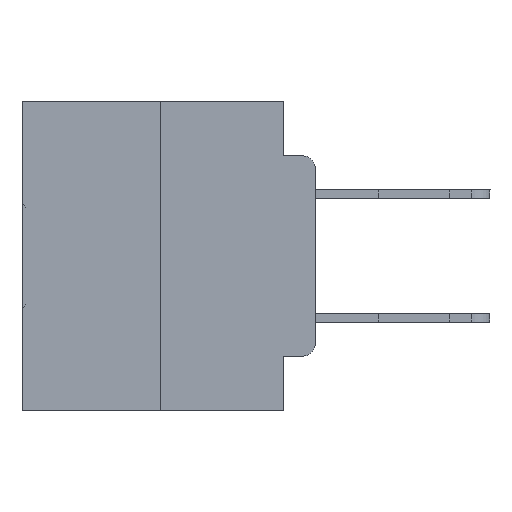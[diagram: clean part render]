
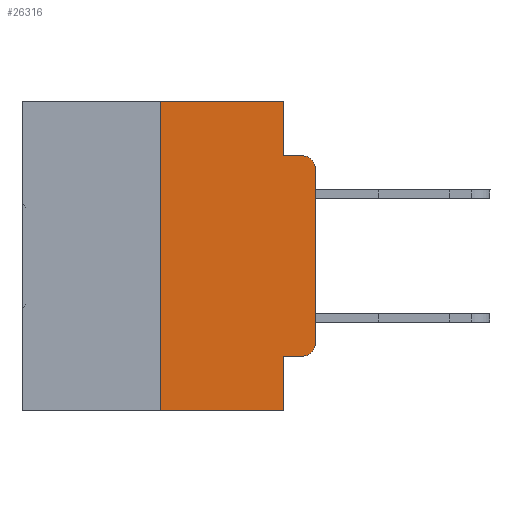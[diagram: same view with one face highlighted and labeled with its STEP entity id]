
A CAD part, left-side view. The second image highlights one B-rep face of the part: STEP entity #26316.
In plain terms, the highlighted planar face has unit normal (-1, 0, 0).
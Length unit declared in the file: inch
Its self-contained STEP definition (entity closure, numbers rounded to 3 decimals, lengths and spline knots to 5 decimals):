
#191 = ORIENTED_EDGE ( 'NONE', *, *, #10974, .T. ) ;
#328 = EDGE_CURVE ( 'NONE', #5537, #6284, #32345, .T. ) ;
#333 = ORIENTED_EDGE ( 'NONE', *, *, #328, .F. ) ;
#639 = CARTESIAN_POINT ( 'NONE',  ( 0., 0., 0. ) ) ;
#1246 = VECTOR ( 'NONE', #32396, 39.37008 ) ;
#1451 = EDGE_CURVE ( 'NONE', #7084, #6441, #4992, .T. ) ;
#1473 = CARTESIAN_POINT ( 'NONE',  ( 0., 0.051, -0.4115 ) ) ;
#1488 = EDGE_CURVE ( 'NONE', #19117, #7084, #26306, .T. ) ;
#1860 = LINE ( 'NONE', #32029, #22420 ) ;
#2245 = VECTOR ( 'NONE', #16539, 39.37008 ) ;
#3180 = DIRECTION ( 'NONE',  ( 0., 0., -1. ) ) ;
#4992 = LINE ( 'NONE', #639, #22798 ) ;
#5026 = EDGE_CURVE ( 'NONE', #6441, #25924, #17452, .T. ) ;
#5537 = VERTEX_POINT ( 'NONE', #14257 ) ;
#5823 = DIRECTION ( 'NONE',  ( 0., 0., 1. ) ) ;
#5964 = LINE ( 'NONE', #24060, #26525 ) ;
#6284 = VERTEX_POINT ( 'NONE', #23575 ) ;
#6441 = VERTEX_POINT ( 'NONE', #29427 ) ;
#6510 = CARTESIAN_POINT ( 'NONE',  ( 0., 0.051, 0. ) ) ;
#7084 = VERTEX_POINT ( 'NONE', #23832 ) ;
#7607 = FACE_OUTER_BOUND ( 'NONE', #13161, .T. ) ;
#7897 = DIRECTION ( 'NONE',  ( 0., -1., 0. ) ) ;
#8152 = CARTESIAN_POINT ( 'NONE',  ( 0., 0.02, -0.3915 ) ) ;
#9524 = DIRECTION ( 'NONE',  ( 0., 0., -1. ) ) ;
#10262 = ORIENTED_EDGE ( 'NONE', *, *, #20951, .T. ) ;
#10974 = EDGE_CURVE ( 'NONE', #5537, #23899, #1860, .T. ) ;
#12241 = VECTOR ( 'NONE', #24153, 39.37008 ) ;
#12527 = LINE ( 'NONE', #1473, #2245 ) ;
#12942 = AXIS2_PLACEMENT_3D ( 'NONE', #8152, #18645, #16030 ) ;
#13098 = ORIENTED_EDGE ( 'NONE', *, *, #5026, .T. ) ;
#13161 = EDGE_LOOP ( 'NONE', ( #13974, #13098, #29983, #25853, #30564, #333, #191, #24889, #10262, #20407 ) ) ;
#13367 = CARTESIAN_POINT ( 'NONE',  ( 0., 0.473, 0. ) ) ;
#13407 = AXIS2_PLACEMENT_3D ( 'NONE', #13367, #25927, #3180 ) ;
#13681 = VERTEX_POINT ( 'NONE', #15306 ) ;
#13692 = PLANE ( 'NONE',  #13407 ) ;
#13974 = ORIENTED_EDGE ( 'NONE', *, *, #1451, .T. ) ;
#14257 = CARTESIAN_POINT ( 'NONE',  ( 0., 0.25, -0.5 ) ) ;
#14333 = CARTESIAN_POINT ( 'NONE',  ( 0., 0.02, -0.4115 ) ) ;
#15172 = CARTESIAN_POINT ( 'NONE',  ( 0., 0.051, -0.0885 ) ) ;
#15306 = CARTESIAN_POINT ( 'NONE',  ( 0., 0.051, -0.4115 ) ) ;
#15816 = VERTEX_POINT ( 'NONE', #6510 ) ;
#16030 = DIRECTION ( 'NONE',  ( 0., 0., -1. ) ) ;
#16056 = LINE ( 'NONE', #23054, #20396 ) ;
#16539 = DIRECTION ( 'NONE',  ( 0., -1., 0. ) ) ;
#17262 = EDGE_CURVE ( 'NONE', #6284, #15816, #23765, .T. ) ;
#17452 = CIRCLE ( 'NONE', #23600, 0.02 ) ;
#17694 = EDGE_CURVE ( 'NONE', #13681, #23899, #5964, .T. ) ;
#17931 = CARTESIAN_POINT ( 'NONE',  ( 0., 0.051, -0.5 ) ) ;
#17984 = VERTEX_POINT ( 'NONE', #15172 ) ;
#18645 = DIRECTION ( 'NONE',  ( -1., 0., 0. ) ) ;
#18948 = LINE ( 'NONE', #31442, #12241 ) ;
#19117 = VERTEX_POINT ( 'NONE', #14333 ) ;
#19669 = CARTESIAN_POINT ( 'NONE',  ( 0., 0.02, -0.0885 ) ) ;
#20396 = VECTOR ( 'NONE', #7897, 39.37008 ) ;
#20407 = ORIENTED_EDGE ( 'NONE', *, *, #1488, .T. ) ;
#20951 = EDGE_CURVE ( 'NONE', #13681, #19117, #12527, .T. ) ;
#20970 = DIRECTION ( 'NONE',  ( 0., 0., 1. ) ) ;
#22317 = EDGE_CURVE ( 'NONE', #15816, #17984, #18948, .T. ) ;
#22420 = VECTOR ( 'NONE', #29818, 39.37008 ) ;
#22798 = VECTOR ( 'NONE', #5823, 39.37008 ) ;
#23054 = CARTESIAN_POINT ( 'NONE',  ( 0., 0.051, -0.0885 ) ) ;
#23575 = CARTESIAN_POINT ( 'NONE',  ( 0., 0.25, 0. ) ) ;
#23600 = AXIS2_PLACEMENT_3D ( 'NONE', #24635, #32599, #9524 ) ;
#23765 = LINE ( 'NONE', #32628, #1246 ) ;
#23832 = CARTESIAN_POINT ( 'NONE',  ( 0., 0., -0.3915 ) ) ;
#23899 = VERTEX_POINT ( 'NONE', #17931 ) ;
#24060 = CARTESIAN_POINT ( 'NONE',  ( 0., 0.051, 0. ) ) ;
#24153 = DIRECTION ( 'NONE',  ( 0., 0., -1. ) ) ;
#24439 = VECTOR ( 'NONE', #20970, 39.37008 ) ;
#24635 = CARTESIAN_POINT ( 'NONE',  ( 0., 0.02, -0.1085 ) ) ;
#24889 = ORIENTED_EDGE ( 'NONE', *, *, #17694, .F. ) ;
#25110 = EDGE_CURVE ( 'NONE', #17984, #25924, #16056, .T. ) ;
#25853 = ORIENTED_EDGE ( 'NONE', *, *, #22317, .F. ) ;
#25924 = VERTEX_POINT ( 'NONE', #19669 ) ;
#25927 = DIRECTION ( 'NONE',  ( 1., 0., 0. ) ) ;
#26128 = CARTESIAN_POINT ( 'NONE',  ( 0., 0.25, 0. ) ) ;
#26306 = CIRCLE ( 'NONE', #12942, 0.02 ) ;
#26316 = ADVANCED_FACE ( 'NONE', ( #7607 ), #13692, .F. ) ;
#26525 = VECTOR ( 'NONE', #28719, 39.37008 ) ;
#28719 = DIRECTION ( 'NONE',  ( 0., 0., -1. ) ) ;
#29427 = CARTESIAN_POINT ( 'NONE',  ( 0., 0., -0.1085 ) ) ;
#29818 = DIRECTION ( 'NONE',  ( 0., -1., 0. ) ) ;
#29983 = ORIENTED_EDGE ( 'NONE', *, *, #25110, .F. ) ;
#30564 = ORIENTED_EDGE ( 'NONE', *, *, #17262, .F. ) ;
#31442 = CARTESIAN_POINT ( 'NONE',  ( 0., 0.051, 0. ) ) ;
#32029 = CARTESIAN_POINT ( 'NONE',  ( 0., 0.473, -0.5 ) ) ;
#32345 = LINE ( 'NONE', #26128, #24439 ) ;
#32396 = DIRECTION ( 'NONE',  ( 0., -1., 0. ) ) ;
#32599 = DIRECTION ( 'NONE',  ( -1., 0., 0. ) ) ;
#32628 = CARTESIAN_POINT ( 'NONE',  ( 0., 0.473, 0. ) ) ;
